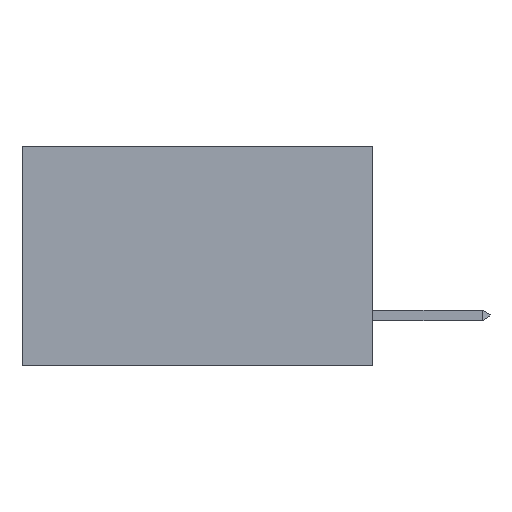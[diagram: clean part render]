
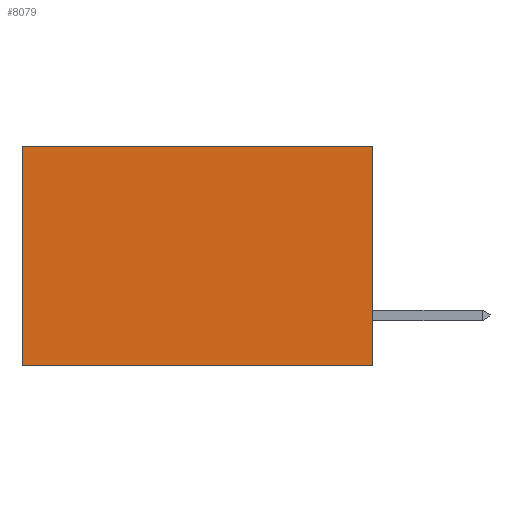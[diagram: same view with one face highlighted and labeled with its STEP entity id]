
A CAD part, left-side view. The second image highlights one B-rep face of the part: STEP entity #8079.
In plain terms, the highlighted planar face has unit normal (-1, 0, 0).
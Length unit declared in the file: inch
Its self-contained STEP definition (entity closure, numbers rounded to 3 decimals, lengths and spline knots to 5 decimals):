
#53 = CARTESIAN_POINT ( 'NONE',  ( 0.277, 0., -0.37 ) ) ;
#410 = PLANE ( 'NONE',  #11753 ) ;
#1054 = DIRECTION ( 'NONE',  ( 0., 1., 0. ) ) ;
#1194 = VECTOR ( 'NONE', #1054, 39.37008 ) ;
#2010 = CARTESIAN_POINT ( 'NONE',  ( 0.277, 0.59, -0.37 ) ) ;
#2030 = EDGE_CURVE ( 'NONE', #5714, #11652, #2894, .T. ) ;
#2168 = VERTEX_POINT ( 'NONE', #7614 ) ;
#2796 = DIRECTION ( 'NONE',  ( 1., 0., 0. ) ) ;
#2821 = EDGE_CURVE ( 'NONE', #3315, #11652, #4273, .T. ) ;
#2894 = LINE ( 'NONE', #2010, #5505 ) ;
#2896 = CARTESIAN_POINT ( 'NONE',  ( 0.277, 0., -0.37 ) ) ;
#3315 = VERTEX_POINT ( 'NONE', #9999 ) ;
#4124 = ORIENTED_EDGE ( 'NONE', *, *, #2030, .T. ) ;
#4273 = LINE ( 'NONE', #53, #1194 ) ;
#5298 = EDGE_LOOP ( 'NONE', ( #4124, #7893, #6797, #10372 ) ) ;
#5505 = VECTOR ( 'NONE', #9715, 39.37008 ) ;
#5511 = CARTESIAN_POINT ( 'NONE',  ( 0.277, 0., 0. ) ) ;
#5714 = VERTEX_POINT ( 'NONE', #7968 ) ;
#5839 = LINE ( 'NONE', #5511, #10676 ) ;
#6588 = DIRECTION ( 'NONE',  ( 0., 1., 0. ) ) ;
#6797 = ORIENTED_EDGE ( 'NONE', *, *, #10068, .F. ) ;
#7614 = CARTESIAN_POINT ( 'NONE',  ( 0.277, 0., 0. ) ) ;
#7893 = ORIENTED_EDGE ( 'NONE', *, *, #2821, .F. ) ;
#7968 = CARTESIAN_POINT ( 'NONE',  ( 0.277, 0.59, 0. ) ) ;
#8079 = ADVANCED_FACE ( 'NONE', ( #12062 ), #410, .F. ) ;
#8463 = VECTOR ( 'NONE', #12371, 39.37008 ) ;
#8800 = LINE ( 'NONE', #2896, #8463 ) ;
#9170 = CARTESIAN_POINT ( 'NONE',  ( 0.277, 0., -0.37 ) ) ;
#9715 = DIRECTION ( 'NONE',  ( 0., 0., -1. ) ) ;
#9999 = CARTESIAN_POINT ( 'NONE',  ( 0.277, 0., -0.37 ) ) ;
#10068 = EDGE_CURVE ( 'NONE', #2168, #3315, #8800, .T. ) ;
#10218 = DIRECTION ( 'NONE',  ( 0., 0., -1. ) ) ;
#10372 = ORIENTED_EDGE ( 'NONE', *, *, #12907, .T. ) ;
#10676 = VECTOR ( 'NONE', #6588, 39.37008 ) ;
#11652 = VERTEX_POINT ( 'NONE', #12790 ) ;
#11753 = AXIS2_PLACEMENT_3D ( 'NONE', #9170, #2796, #10218 ) ;
#12062 = FACE_OUTER_BOUND ( 'NONE', #5298, .T. ) ;
#12371 = DIRECTION ( 'NONE',  ( 0., 0., -1. ) ) ;
#12790 = CARTESIAN_POINT ( 'NONE',  ( 0.277, 0.59, -0.37 ) ) ;
#12907 = EDGE_CURVE ( 'NONE', #2168, #5714, #5839, .T. ) ;
